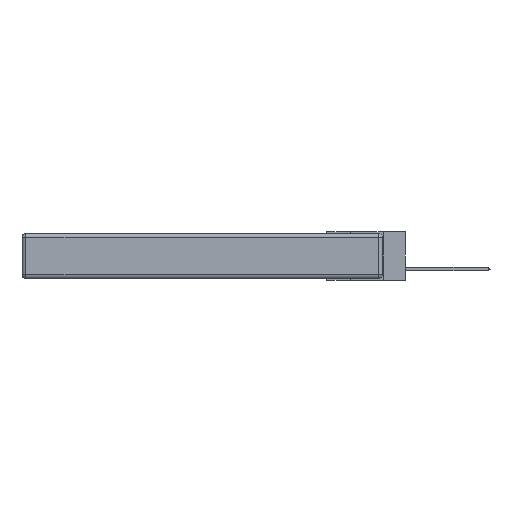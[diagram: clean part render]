
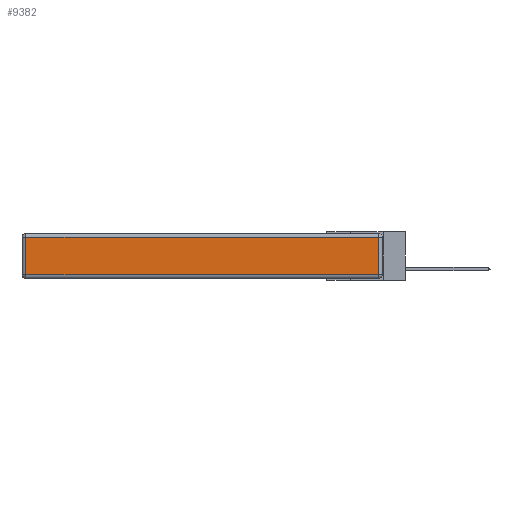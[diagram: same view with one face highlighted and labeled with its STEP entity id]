
A CAD part, left-side view. The second image highlights one B-rep face of the part: STEP entity #9382.
In plain terms, the highlighted planar face has unit normal (-1, 0, 0).
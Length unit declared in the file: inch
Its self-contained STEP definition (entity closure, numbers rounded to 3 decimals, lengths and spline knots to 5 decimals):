
#707 = CARTESIAN_POINT ( 'NONE',  ( 0., 2.72, -0.313 ) ) ;
#732 = VERTEX_POINT ( 'NONE', #8638 ) ;
#777 = LINE ( 'NONE', #3565, #2769 ) ;
#812 = VECTOR ( 'NONE', #8438, 39.37008 ) ;
#899 = EDGE_LOOP ( 'NONE', ( #7217, #8296, #3593, #2502 ) ) ;
#1199 = AXIS2_PLACEMENT_3D ( 'NONE', #9494, #7641, #3670 ) ;
#2219 = CARTESIAN_POINT ( 'NONE',  ( 0., 2.72, -0.03 ) ) ;
#2502 = ORIENTED_EDGE ( 'NONE', *, *, #4428, .T. ) ;
#2547 = CARTESIAN_POINT ( 'NONE',  ( 0., 2.75, -0.03 ) ) ;
#2769 = VECTOR ( 'NONE', #12354, 39.37008 ) ;
#3052 = VECTOR ( 'NONE', #5389, 39.37008 ) ;
#3565 = CARTESIAN_POINT ( 'NONE',  ( 0., 0.03, -0.343 ) ) ;
#3593 = ORIENTED_EDGE ( 'NONE', *, *, #12047, .T. ) ;
#3623 = VERTEX_POINT ( 'NONE', #707 ) ;
#3670 = DIRECTION ( 'NONE',  ( 0., 0., 1. ) ) ;
#3778 = CARTESIAN_POINT ( 'NONE',  ( 0., 2.72, -0.343 ) ) ;
#3838 = VECTOR ( 'NONE', #5776, 39.37008 ) ;
#4428 = EDGE_CURVE ( 'NONE', #11790, #3623, #12550, .T. ) ;
#5018 = EDGE_CURVE ( 'NONE', #732, #6311, #777, .T. ) ;
#5389 = DIRECTION ( 'NONE',  ( 0., -1., 0. ) ) ;
#5776 = DIRECTION ( 'NONE',  ( 0., 0., -1. ) ) ;
#6282 = LINE ( 'NONE', #11211, #3052 ) ;
#6311 = VERTEX_POINT ( 'NONE', #11472 ) ;
#7217 = ORIENTED_EDGE ( 'NONE', *, *, #7813, .T. ) ;
#7641 = DIRECTION ( 'NONE',  ( -1., 0., 0. ) ) ;
#7813 = EDGE_CURVE ( 'NONE', #3623, #732, #6282, .T. ) ;
#8296 = ORIENTED_EDGE ( 'NONE', *, *, #5018, .T. ) ;
#8310 = LINE ( 'NONE', #2547, #812 ) ;
#8438 = DIRECTION ( 'NONE',  ( 0., 1., 0. ) ) ;
#8638 = CARTESIAN_POINT ( 'NONE',  ( 0., 0.03, -0.313 ) ) ;
#8648 = PLANE ( 'NONE',  #1199 ) ;
#9382 = ADVANCED_FACE ( 'NONE', ( #10792 ), #8648, .T. ) ;
#9494 = CARTESIAN_POINT ( 'NONE',  ( 0., 0., -0.343 ) ) ;
#10792 = FACE_OUTER_BOUND ( 'NONE', #899, .T. ) ;
#11211 = CARTESIAN_POINT ( 'NONE',  ( 0., 0., -0.313 ) ) ;
#11472 = CARTESIAN_POINT ( 'NONE',  ( 0., 0.03, -0.03 ) ) ;
#11790 = VERTEX_POINT ( 'NONE', #2219 ) ;
#12047 = EDGE_CURVE ( 'NONE', #6311, #11790, #8310, .T. ) ;
#12354 = DIRECTION ( 'NONE',  ( 0., 0., 1. ) ) ;
#12550 = LINE ( 'NONE', #3778, #3838 ) ;
